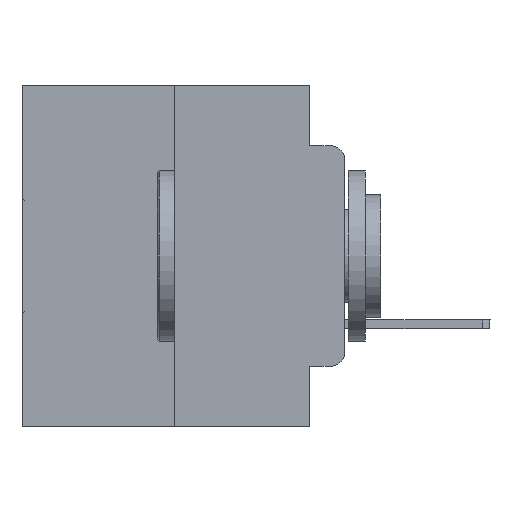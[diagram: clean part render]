
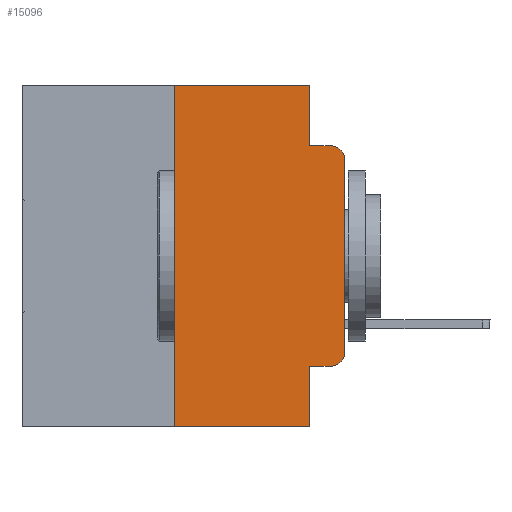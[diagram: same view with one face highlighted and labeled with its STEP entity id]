
A CAD part, left-side view. The second image highlights one B-rep face of the part: STEP entity #15096.
In plain terms, the highlighted planar face has unit normal (-1, 0, 0).
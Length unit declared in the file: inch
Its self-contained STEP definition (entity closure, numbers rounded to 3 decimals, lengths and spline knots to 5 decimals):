
#209 = EDGE_CURVE ( 'NONE', #24243, #24172, #4762, .T. ) ;
#225 = CARTESIAN_POINT ( 'NONE',  ( 0., 0.051, -0.4115 ) ) ;
#1335 = FACE_OUTER_BOUND ( 'NONE', #13261, .T. ) ;
#1375 = ORIENTED_EDGE ( 'NONE', *, *, #22738, .T. ) ;
#1504 = CARTESIAN_POINT ( 'NONE',  ( 0., 0.02, -0.0885 ) ) ;
#2448 = CARTESIAN_POINT ( 'NONE',  ( 0., 0.051, -0.5 ) ) ;
#2569 = ORIENTED_EDGE ( 'NONE', *, *, #5642, .F. ) ;
#2647 = CARTESIAN_POINT ( 'NONE',  ( 0., 0.25, 0. ) ) ;
#2717 = DIRECTION ( 'NONE',  ( -1., 0., 0. ) ) ;
#2744 = EDGE_CURVE ( 'NONE', #24243, #27391, #7019, .T. ) ;
#2807 = EDGE_CURVE ( 'NONE', #21835, #23137, #16696, .T. ) ;
#3185 = ORIENTED_EDGE ( 'NONE', *, *, #3706, .F. ) ;
#3232 = AXIS2_PLACEMENT_3D ( 'NONE', #21253, #19352, #9971 ) ;
#3396 = PLANE ( 'NONE',  #3232 ) ;
#3615 = VERTEX_POINT ( 'NONE', #28416 ) ;
#3668 = ORIENTED_EDGE ( 'NONE', *, *, #14334, .T. ) ;
#3691 = VERTEX_POINT ( 'NONE', #25244 ) ;
#3706 = EDGE_CURVE ( 'NONE', #7396, #3691, #27589, .T. ) ;
#4713 = ORIENTED_EDGE ( 'NONE', *, *, #2744, .F. ) ;
#4763 = ORIENTED_EDGE ( 'NONE', *, *, #2807, .T. ) ;
#4762 = LINE ( 'NONE', #12030, #18451 ) ;
#4798 = LINE ( 'NONE', #225, #19231 ) ;
#5074 = CIRCLE ( 'NONE', #8325, 0.02 ) ;
#5642 = EDGE_CURVE ( 'NONE', #27391, #7396, #6731, .T. ) ;
#6731 = LINE ( 'NONE', #7562, #17284 ) ;
#6844 = VERTEX_POINT ( 'NONE', #22403 ) ;
#7019 = LINE ( 'NONE', #15950, #7759 ) ;
#7396 = VERTEX_POINT ( 'NONE', #25550 ) ;
#7562 = CARTESIAN_POINT ( 'NONE',  ( 0., 0.473, 0. ) ) ;
#7759 = VECTOR ( 'NONE', #16232, 39.37008 ) ;
#8008 = CARTESIAN_POINT ( 'NONE',  ( 0., 0.051, -0.0885 ) ) ;
#8171 = VECTOR ( 'NONE', #24654, 39.37008 ) ;
#8325 = AXIS2_PLACEMENT_3D ( 'NONE', #9313, #2717, #25123 ) ;
#9313 = CARTESIAN_POINT ( 'NONE',  ( 0., 0.02, -0.3915 ) ) ;
#9425 = DIRECTION ( 'NONE',  ( 0., -1., 0. ) ) ;
#9849 = CARTESIAN_POINT ( 'NONE',  ( 0., 0.051, 0. ) ) ;
#9971 = DIRECTION ( 'NONE',  ( 0., 0., -1. ) ) ;
#10152 = VECTOR ( 'NONE', #25385, 39.37008 ) ;
#11102 = ORIENTED_EDGE ( 'NONE', *, *, #14092, .F. ) ;
#12008 = CARTESIAN_POINT ( 'NONE',  ( 0., 0., -0.1085 ) ) ;
#12030 = CARTESIAN_POINT ( 'NONE',  ( 0., 0.473, -0.5 ) ) ;
#12062 = VERTEX_POINT ( 'NONE', #22124 ) ;
#12249 = DIRECTION ( 'NONE',  ( 0., 0., -1. ) ) ;
#13261 = EDGE_LOOP ( 'NONE', ( #1375, #4763, #11102, #3185, #2569, #4713, #20734, #15893, #18558, #3668 ) ) ;
#13323 = CARTESIAN_POINT ( 'NONE',  ( 0., 0.051, 0. ) ) ;
#13377 = EDGE_CURVE ( 'NONE', #12062, #24172, #19790, .T. ) ;
#13562 = DIRECTION ( 'NONE',  ( 0., -1., 0. ) ) ;
#14092 = EDGE_CURVE ( 'NONE', #3691, #23137, #19282, .T. ) ;
#14334 = EDGE_CURVE ( 'NONE', #6844, #3615, #5074, .T. ) ;
#14738 = DIRECTION ( 'NONE',  ( -1., 0., 0. ) ) ;
#14821 = CARTESIAN_POINT ( 'NONE',  ( 0., 0.25, -0.5 ) ) ;
#15096 = ADVANCED_FACE ( 'NONE', ( #1335 ), #3396, .F. ) ;
#15893 = ORIENTED_EDGE ( 'NONE', *, *, #13377, .F. ) ;
#15950 = CARTESIAN_POINT ( 'NONE',  ( 0., 0.25, 0. ) ) ;
#16232 = DIRECTION ( 'NONE',  ( 0., 0., 1. ) ) ;
#16696 = CIRCLE ( 'NONE', #24152, 0.02 ) ;
#17284 = VECTOR ( 'NONE', #20349, 39.37008 ) ;
#17500 = EDGE_CURVE ( 'NONE', #12062, #6844, #4798, .T. ) ;
#17620 = LINE ( 'NONE', #26859, #8171 ) ;
#17722 = DIRECTION ( 'NONE',  ( 0., 0., -1. ) ) ;
#18451 = VECTOR ( 'NONE', #9425, 39.37008 ) ;
#18558 = ORIENTED_EDGE ( 'NONE', *, *, #17500, .T. ) ;
#19231 = VECTOR ( 'NONE', #13562, 39.37008 ) ;
#19282 = LINE ( 'NONE', #8008, #21420 ) ;
#19352 = DIRECTION ( 'NONE',  ( 1., 0., 0. ) ) ;
#19790 = LINE ( 'NONE', #13323, #25192 ) ;
#20349 = DIRECTION ( 'NONE',  ( 0., -1., 0. ) ) ;
#20734 = ORIENTED_EDGE ( 'NONE', *, *, #209, .T. ) ;
#21253 = CARTESIAN_POINT ( 'NONE',  ( 0., 0.473, 0. ) ) ;
#21420 = VECTOR ( 'NONE', #25869, 39.37008 ) ;
#21835 = VERTEX_POINT ( 'NONE', #12008 ) ;
#22124 = CARTESIAN_POINT ( 'NONE',  ( 0., 0.051, -0.4115 ) ) ;
#22403 = CARTESIAN_POINT ( 'NONE',  ( 0., 0.02, -0.4115 ) ) ;
#22738 = EDGE_CURVE ( 'NONE', #3615, #21835, #17620, .T. ) ;
#23137 = VERTEX_POINT ( 'NONE', #1504 ) ;
#23388 = CARTESIAN_POINT ( 'NONE',  ( 0., 0.02, -0.1085 ) ) ;
#24152 = AXIS2_PLACEMENT_3D ( 'NONE', #23388, #14738, #12249 ) ;
#24172 = VERTEX_POINT ( 'NONE', #2448 ) ;
#24243 = VERTEX_POINT ( 'NONE', #14821 ) ;
#24654 = DIRECTION ( 'NONE',  ( 0., 0., 1. ) ) ;
#25123 = DIRECTION ( 'NONE',  ( 0., 0., -1. ) ) ;
#25192 = VECTOR ( 'NONE', #17722, 39.37008 ) ;
#25244 = CARTESIAN_POINT ( 'NONE',  ( 0., 0.051, -0.0885 ) ) ;
#25385 = DIRECTION ( 'NONE',  ( 0., 0., -1. ) ) ;
#25550 = CARTESIAN_POINT ( 'NONE',  ( 0., 0.051, 0. ) ) ;
#25869 = DIRECTION ( 'NONE',  ( 0., -1., 0. ) ) ;
#26859 = CARTESIAN_POINT ( 'NONE',  ( 0., 0., 0. ) ) ;
#27391 = VERTEX_POINT ( 'NONE', #2647 ) ;
#27589 = LINE ( 'NONE', #9849, #10152 ) ;
#28416 = CARTESIAN_POINT ( 'NONE',  ( 0., 0., -0.3915 ) ) ;
